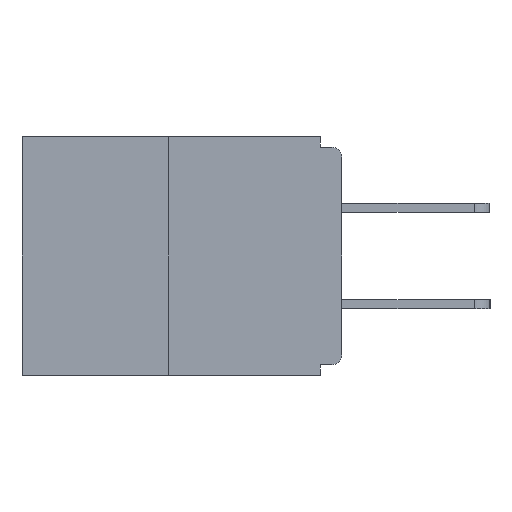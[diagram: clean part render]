
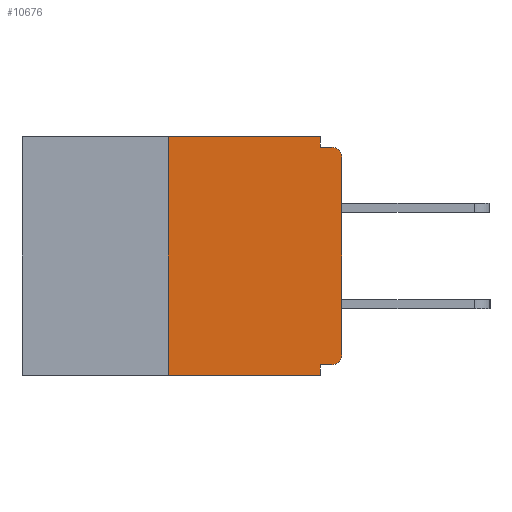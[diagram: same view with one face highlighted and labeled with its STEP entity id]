
A CAD part, left-side view. The second image highlights one B-rep face of the part: STEP entity #10676.
In plain terms, the highlighted planar face has unit normal (-1, 0, 0).
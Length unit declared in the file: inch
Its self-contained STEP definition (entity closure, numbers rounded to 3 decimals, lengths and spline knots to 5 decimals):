
#329 = EDGE_CURVE ( 'NONE', #5672, #19561, #24294, .T. ) ;
#792 = LINE ( 'NONE', #16334, #7076 ) ;
#886 = VERTEX_POINT ( 'NONE', #12032 ) ;
#1645 = CARTESIAN_POINT ( 'NONE',  ( 0., 0.015, -0.015 ) ) ;
#1757 = ORIENTED_EDGE ( 'NONE', *, *, #10704, .T. ) ;
#2313 = VERTEX_POINT ( 'NONE', #7943 ) ;
#2353 = LINE ( 'NONE', #9639, #27495 ) ;
#2697 = ORIENTED_EDGE ( 'NONE', *, *, #5712, .F. ) ;
#3205 = CARTESIAN_POINT ( 'NONE',  ( 0., 0.25, 0. ) ) ;
#3747 = CARTESIAN_POINT ( 'NONE',  ( 0., 0., -0.03 ) ) ;
#3782 = VECTOR ( 'NONE', #10765, 39.37008 ) ;
#3835 = EDGE_CURVE ( 'NONE', #19575, #15135, #25549, .T. ) ;
#4384 = VECTOR ( 'NONE', #14330, 39.37008 ) ;
#4466 = CARTESIAN_POINT ( 'NONE',  ( 0., 0.25, -0.343 ) ) ;
#4833 = VECTOR ( 'NONE', #12116, 39.37008 ) ;
#4993 = DIRECTION ( 'NONE',  ( 0., 0., -1. ) ) ;
#5108 = EDGE_CURVE ( 'NONE', #2313, #22150, #25431, .T. ) ;
#5616 = DIRECTION ( 'NONE',  ( 0., 1., 0. ) ) ;
#5618 = VECTOR ( 'NONE', #24455, 39.37008 ) ;
#5672 = VERTEX_POINT ( 'NONE', #3747 ) ;
#5712 = EDGE_CURVE ( 'NONE', #22150, #19352, #26665, .T. ) ;
#6994 = DIRECTION ( 'NONE',  ( -1., 0., 0. ) ) ;
#7030 = CARTESIAN_POINT ( 'NONE',  ( 0., 0.46, 0. ) ) ;
#7076 = VECTOR ( 'NONE', #7828, 39.37008 ) ;
#7828 = DIRECTION ( 'NONE',  ( 0., 0., -1. ) ) ;
#7932 = CARTESIAN_POINT ( 'NONE',  ( 0., 0., -0.015 ) ) ;
#7943 = CARTESIAN_POINT ( 'NONE',  ( 0., 0.015, -0.328 ) ) ;
#8813 = CARTESIAN_POINT ( 'NONE',  ( 0., 0.031, -0.343 ) ) ;
#8931 = CARTESIAN_POINT ( 'NONE',  ( 0., 0.031, -0.328 ) ) ;
#9587 = VECTOR ( 'NONE', #5616, 39.37008 ) ;
#9590 = CARTESIAN_POINT ( 'NONE',  ( 0., 0.031, -0.015 ) ) ;
#9639 = CARTESIAN_POINT ( 'NONE',  ( 0., 0.46, 0. ) ) ;
#10158 = ORIENTED_EDGE ( 'NONE', *, *, #22270, .T. ) ;
#10175 = LINE ( 'NONE', #19269, #3782 ) ;
#10676 = ADVANCED_FACE ( 'NONE', ( #18375 ), #27427, .F. ) ;
#10704 = EDGE_CURVE ( 'NONE', #12036, #5672, #21768, .T. ) ;
#10710 = EDGE_CURVE ( 'NONE', #23556, #19561, #18953, .T. ) ;
#10765 = DIRECTION ( 'NONE',  ( 0., -1., 0. ) ) ;
#11119 = AXIS2_PLACEMENT_3D ( 'NONE', #25398, #27910, #4993 ) ;
#11570 = CARTESIAN_POINT ( 'NONE',  ( 0., 0.25, 0. ) ) ;
#12032 = CARTESIAN_POINT ( 'NONE',  ( 0., 0.031, 0. ) ) ;
#12036 = VERTEX_POINT ( 'NONE', #20345 ) ;
#12116 = DIRECTION ( 'NONE',  ( 0., 0., 1. ) ) ;
#12320 = CARTESIAN_POINT ( 'NONE',  ( 0., 0., -0.328 ) ) ;
#12321 = ORIENTED_EDGE ( 'NONE', *, *, #16434, .F. ) ;
#13580 = CARTESIAN_POINT ( 'NONE',  ( 0., 0.015, -0.03 ) ) ;
#14081 = DIRECTION ( 'NONE',  ( 0., 0., 1. ) ) ;
#14330 = DIRECTION ( 'NONE',  ( 0., -1., 0. ) ) ;
#14941 = ORIENTED_EDGE ( 'NONE', *, *, #18338, .F. ) ;
#15135 = VERTEX_POINT ( 'NONE', #3205 ) ;
#16141 = DIRECTION ( 'NONE',  ( 1., 0., 0. ) ) ;
#16334 = CARTESIAN_POINT ( 'NONE',  ( 0., 0.031, 0. ) ) ;
#16434 = EDGE_CURVE ( 'NONE', #15135, #886, #2353, .T. ) ;
#16819 = CIRCLE ( 'NONE', #11119, 0.015 ) ;
#17245 = AXIS2_PLACEMENT_3D ( 'NONE', #7030, #16141, #22976 ) ;
#18122 = AXIS2_PLACEMENT_3D ( 'NONE', #13580, #6994, #20143 ) ;
#18338 = EDGE_CURVE ( 'NONE', #886, #23556, #792, .T. ) ;
#18375 = FACE_OUTER_BOUND ( 'NONE', #24510, .T. ) ;
#18953 = LINE ( 'NONE', #7932, #4384 ) ;
#19070 = EDGE_CURVE ( 'NONE', #19575, #19352, #10175, .T. ) ;
#19269 = CARTESIAN_POINT ( 'NONE',  ( 0., 0.46, -0.343 ) ) ;
#19352 = VERTEX_POINT ( 'NONE', #25327 ) ;
#19561 = VERTEX_POINT ( 'NONE', #1645 ) ;
#19575 = VERTEX_POINT ( 'NONE', #4466 ) ;
#20047 = ORIENTED_EDGE ( 'NONE', *, *, #5108, .F. ) ;
#20143 = DIRECTION ( 'NONE',  ( 0., 0., -1. ) ) ;
#20272 = ORIENTED_EDGE ( 'NONE', *, *, #10710, .F. ) ;
#20345 = CARTESIAN_POINT ( 'NONE',  ( 0., 0., -0.313 ) ) ;
#20769 = ORIENTED_EDGE ( 'NONE', *, *, #19070, .T. ) ;
#21768 = LINE ( 'NONE', #28619, #4833 ) ;
#22150 = VERTEX_POINT ( 'NONE', #8931 ) ;
#22270 = EDGE_CURVE ( 'NONE', #2313, #12036, #16819, .T. ) ;
#22976 = DIRECTION ( 'NONE',  ( 0., 0., -1. ) ) ;
#23556 = VERTEX_POINT ( 'NONE', #9590 ) ;
#24132 = ORIENTED_EDGE ( 'NONE', *, *, #3835, .F. ) ;
#24294 = CIRCLE ( 'NONE', #18122, 0.015 ) ;
#24455 = DIRECTION ( 'NONE',  ( 0., 0., -1. ) ) ;
#24510 = EDGE_LOOP ( 'NONE', ( #12321, #24132, #20769, #2697, #20047, #10158, #1757, #27442, #20272, #14941 ) ) ;
#25327 = CARTESIAN_POINT ( 'NONE',  ( 0., 0.031, -0.343 ) ) ;
#25398 = CARTESIAN_POINT ( 'NONE',  ( 0., 0.015, -0.313 ) ) ;
#25431 = LINE ( 'NONE', #12320, #9587 ) ;
#25549 = LINE ( 'NONE', #11570, #28627 ) ;
#26665 = LINE ( 'NONE', #8813, #5618 ) ;
#27427 = PLANE ( 'NONE',  #17245 ) ;
#27442 = ORIENTED_EDGE ( 'NONE', *, *, #329, .T. ) ;
#27495 = VECTOR ( 'NONE', #27957, 39.37008 ) ;
#27910 = DIRECTION ( 'NONE',  ( -1., 0., 0. ) ) ;
#27957 = DIRECTION ( 'NONE',  ( 0., -1., 0. ) ) ;
#28619 = CARTESIAN_POINT ( 'NONE',  ( 0., 0., 0. ) ) ;
#28627 = VECTOR ( 'NONE', #14081, 39.37008 ) ;
